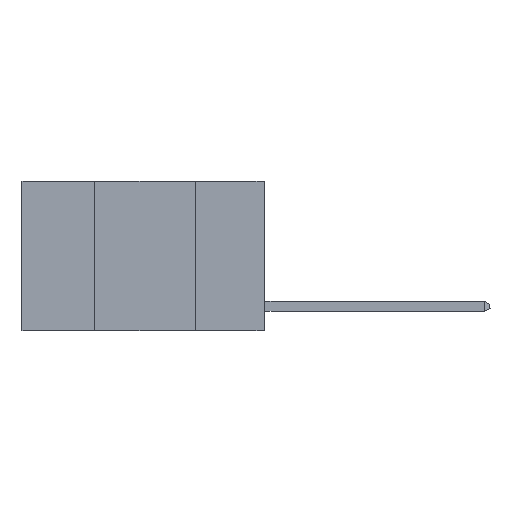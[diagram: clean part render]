
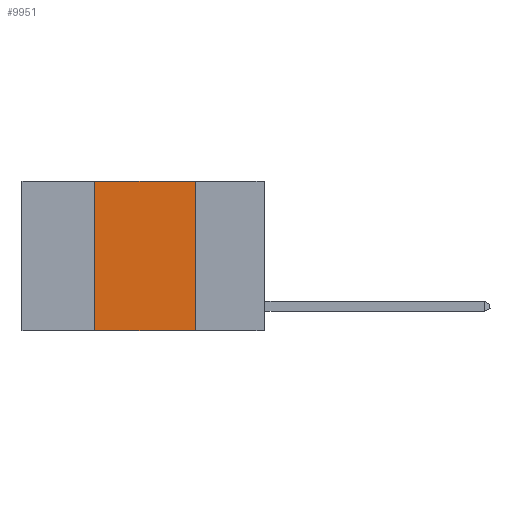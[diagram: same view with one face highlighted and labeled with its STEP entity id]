
A CAD part, left-side view. The second image highlights one B-rep face of the part: STEP entity #9951.
In plain terms, the highlighted planar face has unit normal (-1, 0, 0).
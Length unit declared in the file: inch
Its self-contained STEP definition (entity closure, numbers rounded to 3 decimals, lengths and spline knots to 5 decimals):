
#64 = VERTEX_POINT ( 'NONE', #4159 ) ;
#84 = CARTESIAN_POINT ( 'NONE',  ( 0., 0.42, 0. ) ) ;
#711 = CARTESIAN_POINT ( 'NONE',  ( 0., 0.42, 0. ) ) ;
#1470 = DIRECTION ( 'NONE',  ( 0., 0., -1. ) ) ;
#1693 = VERTEX_POINT ( 'NONE', #8335 ) ;
#1877 = LINE ( 'NONE', #12987, #7109 ) ;
#2052 = CARTESIAN_POINT ( 'NONE',  ( 0., 0.6, -0.37 ) ) ;
#2337 = CARTESIAN_POINT ( 'NONE',  ( 0., 0.17, 0. ) ) ;
#2411 = EDGE_LOOP ( 'NONE', ( #13211, #7776, #7100, #3335 ) ) ;
#2500 = DIRECTION ( 'NONE',  ( 0., -1., 0. ) ) ;
#3335 = ORIENTED_EDGE ( 'NONE', *, *, #4517, .T. ) ;
#4159 = CARTESIAN_POINT ( 'NONE',  ( 0., 0.17, -0.37 ) ) ;
#4442 = DIRECTION ( 'NONE',  ( 0., 0., -1. ) ) ;
#4517 = EDGE_CURVE ( 'NONE', #8961, #64, #7688, .T. ) ;
#4851 = VECTOR ( 'NONE', #7395, 39.37008 ) ;
#4890 = VECTOR ( 'NONE', #13579, 39.37008 ) ;
#4970 = VERTEX_POINT ( 'NONE', #711 ) ;
#5937 = CARTESIAN_POINT ( 'NONE',  ( 0., 0.42, -0.37 ) ) ;
#7100 = ORIENTED_EDGE ( 'NONE', *, *, #12299, .F. ) ;
#7109 = VECTOR ( 'NONE', #2500, 39.37008 ) ;
#7303 = LINE ( 'NONE', #84, #4851 ) ;
#7374 = LINE ( 'NONE', #2337, #11195 ) ;
#7395 = DIRECTION ( 'NONE',  ( 0., 0., 1. ) ) ;
#7595 = EDGE_CURVE ( 'NONE', #4970, #1693, #1877, .T. ) ;
#7629 = AXIS2_PLACEMENT_3D ( 'NONE', #7697, #7740, #1470 ) ;
#7688 = LINE ( 'NONE', #2052, #4890 ) ;
#7697 = CARTESIAN_POINT ( 'NONE',  ( 0., 0.6, 0. ) ) ;
#7740 = DIRECTION ( 'NONE',  ( 1., 0., 0. ) ) ;
#7776 = ORIENTED_EDGE ( 'NONE', *, *, #7595, .F. ) ;
#8335 = CARTESIAN_POINT ( 'NONE',  ( 0., 0.17, 0. ) ) ;
#8961 = VERTEX_POINT ( 'NONE', #5937 ) ;
#9845 = EDGE_CURVE ( 'NONE', #1693, #64, #7374, .T. ) ;
#9951 = ADVANCED_FACE ( 'NONE', ( #11702 ), #11982, .F. ) ;
#11195 = VECTOR ( 'NONE', #4442, 39.37008 ) ;
#11702 = FACE_OUTER_BOUND ( 'NONE', #2411, .T. ) ;
#11982 = PLANE ( 'NONE',  #7629 ) ;
#12299 = EDGE_CURVE ( 'NONE', #8961, #4970, #7303, .T. ) ;
#12987 = CARTESIAN_POINT ( 'NONE',  ( 0., 0.6, 0. ) ) ;
#13211 = ORIENTED_EDGE ( 'NONE', *, *, #9845, .F. ) ;
#13579 = DIRECTION ( 'NONE',  ( 0., -1., 0. ) ) ;
